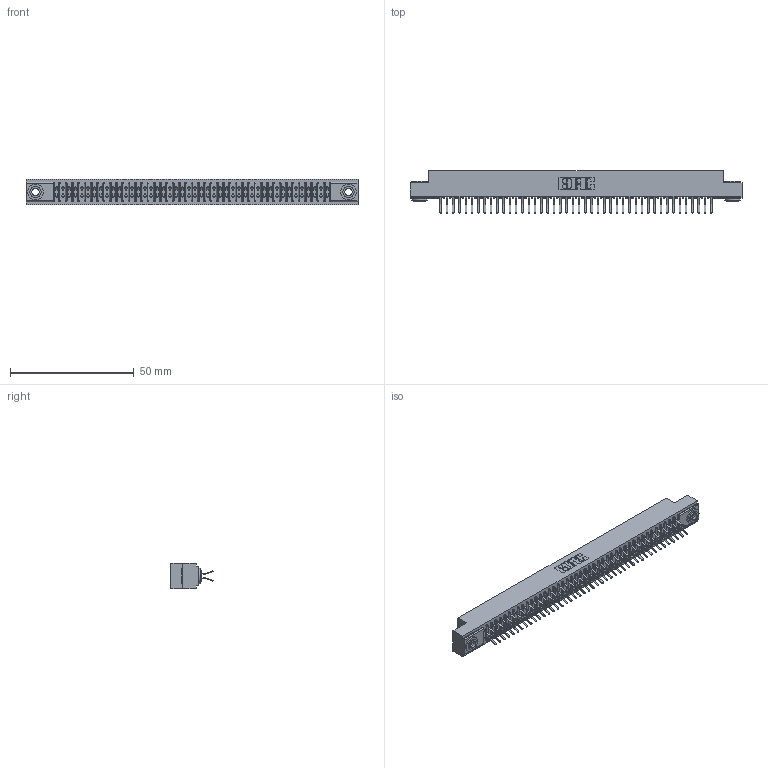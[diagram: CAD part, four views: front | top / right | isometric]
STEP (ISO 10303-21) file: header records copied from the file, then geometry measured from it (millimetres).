
FILE_DESCRIPTION (( 'STEP AP203' ), '1' );
FILE_NAME ('341-088-556-203.STEP', '2018-08-07T23:46:37', ( '' ), ( '' ), 'SwSTEP 2.0', 'SolidWorks 2016', '' );
FILE_SCHEMA (( 'CONFIG_CONTROL_DESIGN' ));
Length unit declared in the file: inch
Products named in the file (4): 345-250-002_345-250-002-102; 341-088-556-203; 341 Part_.156 (3.96) Dia Mounting Holes; 341-292-001_341-292-156
Assembly tree (91 placements, depth 2):
  341-088-556-203
    341 Part_.156 (3.96) Dia Mounting Holes
    341-292-001_341-292-156  x88
    345-250-002_345-250-002-102  x2
Bounding box: 133.99 x 17.07 x 10.16 mm (x, y, z)
Volume: 9925.2 mm3; surface area: 18136.3 mm2
Topology: 91 solids, 91 shells, 6328 faces, 18336 edges, 11894 vertices
Faces by surface type: plane 3612, cylinder 2532, sphere 90, torus 86, cone 8
Entity records: 54188 total; most frequent: CARTESIAN_POINT 8989, ORIENTED_EDGE 8924, DIRECTION 8742, EDGE_CURVE 4462, VECTOR 3592, LINE 3592, VERTEX_POINT 2822, AXIS2_PLACEMENT_3D 2575
